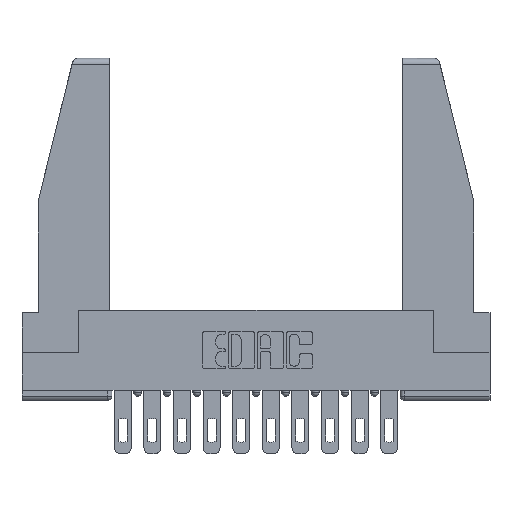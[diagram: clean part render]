
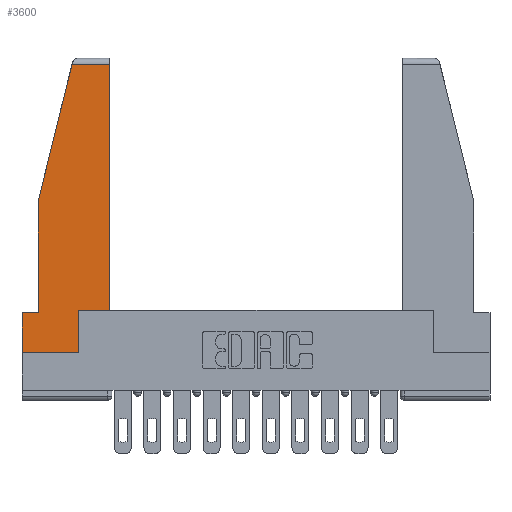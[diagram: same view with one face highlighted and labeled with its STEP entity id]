
A CAD part, top view. The second image highlights one B-rep face of the part: STEP entity #3600.
In plain terms, the highlighted planar face has unit normal (0, 0, 1).
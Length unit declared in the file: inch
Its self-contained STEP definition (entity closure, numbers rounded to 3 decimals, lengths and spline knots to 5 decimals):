
#119 = CARTESIAN_POINT ( 'NONE',  ( 0.271, 1.55, 0. ) ) ;
#463 = ORIENTED_EDGE ( 'NONE', *, *, #9780, .T. ) ;
#588 = CARTESIAN_POINT ( 'NONE',  ( 0., 0., 0. ) ) ;
#778 = CARTESIAN_POINT ( 'NONE',  ( 0., 0.21, 0. ) ) ;
#840 = LINE ( 'NONE', #11514, #5860 ) ;
#859 = EDGE_CURVE ( 'NONE', #5648, #12797, #9394, .T. ) ;
#933 = DIRECTION ( 'NONE',  ( 0., 1., 0. ) ) ;
#956 = DIRECTION ( 'NONE',  ( -1., 0., 0. ) ) ;
#1006 = VECTOR ( 'NONE', #11512, 39.37008 ) ;
#1519 = VECTOR ( 'NONE', #14201, 39.37008 ) ;
#2552 = ORIENTED_EDGE ( 'NONE', *, *, #13962, .T. ) ;
#2888 = EDGE_CURVE ( 'NONE', #8162, #11591, #840, .T. ) ;
#3106 = CARTESIAN_POINT ( 'NONE',  ( 0.2636, 1.52, 0. ) ) ;
#3389 = VERTEX_POINT ( 'NONE', #14951 ) ;
#3495 = LINE ( 'NONE', #12908, #4214 ) ;
#3600 = ADVANCED_FACE ( 'NONE', ( #13363 ), #9979, .T. ) ;
#4053 = EDGE_CURVE ( 'NONE', #13699, #8162, #11287, .T. ) ;
#4214 = VECTOR ( 'NONE', #933, 39.37008 ) ;
#4352 = VERTEX_POINT ( 'NONE', #6180 ) ;
#4473 = CARTESIAN_POINT ( 'NONE',  ( 0.461, 1.52, 0. ) ) ;
#4536 = DIRECTION ( 'NONE',  ( 1., 0., 0. ) ) ;
#4546 = VECTOR ( 'NONE', #8694, 39.37008 ) ;
#4633 = CARTESIAN_POINT ( 'NONE',  ( 0.086, 0.8, 0. ) ) ;
#4993 = LINE ( 'NONE', #778, #5670 ) ;
#5049 = LINE ( 'NONE', #14407, #4546 ) ;
#5315 = ORIENTED_EDGE ( 'NONE', *, *, #2888, .T. ) ;
#5648 = VERTEX_POINT ( 'NONE', #4473 ) ;
#5670 = VECTOR ( 'NONE', #14843, 39.37008 ) ;
#5716 = ORIENTED_EDGE ( 'NONE', *, *, #9173, .T. ) ;
#5860 = VECTOR ( 'NONE', #12975, 39.37008 ) ;
#5863 = CARTESIAN_POINT ( 'NONE',  ( 0.297, 0.223, 0. ) ) ;
#6180 = CARTESIAN_POINT ( 'NONE',  ( 0.461, 0.223, 0. ) ) ;
#6736 = DIRECTION ( 'NONE',  ( 1., 0., 0. ) ) ;
#6899 = CARTESIAN_POINT ( 'NONE',  ( 0.297, 0.223, 0. ) ) ;
#7107 = VECTOR ( 'NONE', #13720, 39.37008 ) ;
#7234 = ORIENTED_EDGE ( 'NONE', *, *, #4053, .T. ) ;
#7464 = EDGE_CURVE ( 'NONE', #4352, #5648, #3495, .T. ) ;
#7899 = DIRECTION ( 'NONE',  ( 0., 0., 1. ) ) ;
#8162 = VERTEX_POINT ( 'NONE', #11047 ) ;
#8640 = EDGE_CURVE ( 'NONE', #12225, #3389, #4993, .T. ) ;
#8694 = DIRECTION ( 'NONE',  ( 0., -1., 0. ) ) ;
#8738 = CARTESIAN_POINT ( 'NONE',  ( 0., 0., 0. ) ) ;
#8954 = ORIENTED_EDGE ( 'NONE', *, *, #15133, .T. ) ;
#8968 = CARTESIAN_POINT ( 'NONE',  ( 0., 0., 0. ) ) ;
#9173 = EDGE_CURVE ( 'NONE', #3389, #13699, #13890, .T. ) ;
#9203 = VERTEX_POINT ( 'NONE', #4633 ) ;
#9214 = AXIS2_PLACEMENT_3D ( 'NONE', #8968, #7899, #6736 ) ;
#9277 = CARTESIAN_POINT ( 'NONE',  ( 0., 0.21, 0. ) ) ;
#9394 = LINE ( 'NONE', #10470, #14764 ) ;
#9739 = ORIENTED_EDGE ( 'NONE', *, *, #859, .T. ) ;
#9780 = EDGE_CURVE ( 'NONE', #12797, #9203, #11957, .T. ) ;
#9979 = PLANE ( 'NONE',  #9214 ) ;
#10470 = CARTESIAN_POINT ( 'NONE',  ( 0., 1.52, 0. ) ) ;
#10499 = ORIENTED_EDGE ( 'NONE', *, *, #8640, .T. ) ;
#10951 = CARTESIAN_POINT ( 'NONE',  ( 0.086, 0.21, 0. ) ) ;
#11047 = CARTESIAN_POINT ( 'NONE',  ( 0.297, 0., 0. ) ) ;
#11206 = EDGE_LOOP ( 'NONE', ( #11418, #9739, #463, #2552, #10499, #5716, #7234, #5315, #8954 ) ) ;
#11287 = LINE ( 'NONE', #8738, #7107 ) ;
#11418 = ORIENTED_EDGE ( 'NONE', *, *, #7464, .T. ) ;
#11512 = DIRECTION ( 'NONE',  ( 0., -1., 0. ) ) ;
#11514 = CARTESIAN_POINT ( 'NONE',  ( 0.297, 0., 0. ) ) ;
#11570 = LINE ( 'NONE', #5863, #15192 ) ;
#11591 = VERTEX_POINT ( 'NONE', #6899 ) ;
#11957 = LINE ( 'NONE', #119, #1519 ) ;
#12225 = VERTEX_POINT ( 'NONE', #10951 ) ;
#12797 = VERTEX_POINT ( 'NONE', #3106 ) ;
#12908 = CARTESIAN_POINT ( 'NONE',  ( 0.461, 0.223, 0. ) ) ;
#12975 = DIRECTION ( 'NONE',  ( 0., 1., 0. ) ) ;
#13363 = FACE_OUTER_BOUND ( 'NONE', #11206, .T. ) ;
#13699 = VERTEX_POINT ( 'NONE', #588 ) ;
#13720 = DIRECTION ( 'NONE',  ( 1., 0., 0. ) ) ;
#13890 = LINE ( 'NONE', #9277, #1006 ) ;
#13962 = EDGE_CURVE ( 'NONE', #9203, #12225, #5049, .T. ) ;
#14201 = DIRECTION ( 'NONE',  ( -0.239, -0.971, 0. ) ) ;
#14407 = CARTESIAN_POINT ( 'NONE',  ( 0.086, 0.8, 0. ) ) ;
#14764 = VECTOR ( 'NONE', #956, 39.37008 ) ;
#14843 = DIRECTION ( 'NONE',  ( -1., 0., 0. ) ) ;
#14951 = CARTESIAN_POINT ( 'NONE',  ( 0., 0.21, 0. ) ) ;
#15133 = EDGE_CURVE ( 'NONE', #11591, #4352, #11570, .T. ) ;
#15192 = VECTOR ( 'NONE', #4536, 39.37008 ) ;
